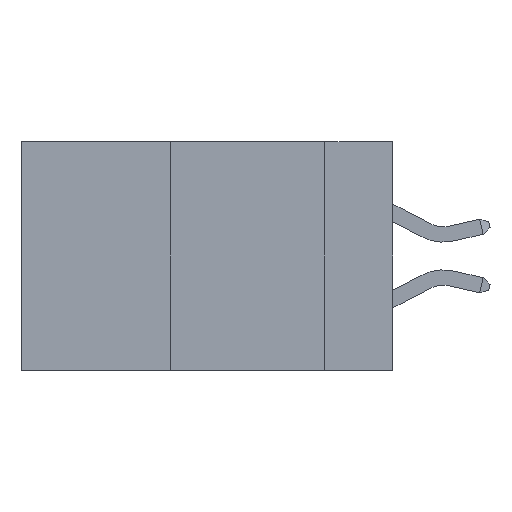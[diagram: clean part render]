
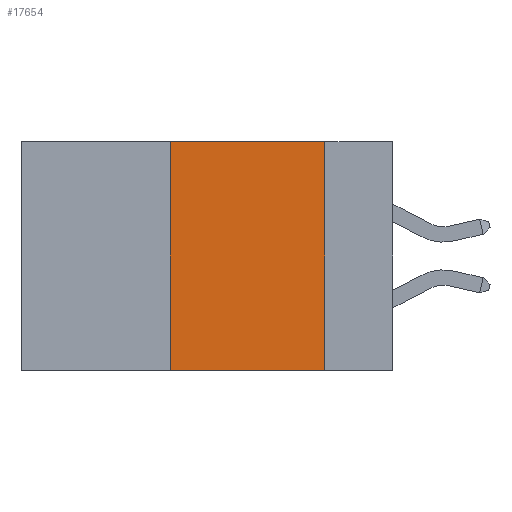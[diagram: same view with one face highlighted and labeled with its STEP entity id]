
A CAD part, left-side view. The second image highlights one B-rep face of the part: STEP entity #17654.
In plain terms, the highlighted planar face has unit normal (-1, 0, 0).
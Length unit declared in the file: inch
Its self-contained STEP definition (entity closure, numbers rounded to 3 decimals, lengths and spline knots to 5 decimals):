
#61 = VECTOR ( 'NONE', #3347, 39.37008 ) ;
#445 = VERTEX_POINT ( 'NONE', #15771 ) ;
#2570 = LINE ( 'NONE', #3486, #11420 ) ;
#2935 = LINE ( 'NONE', #18096, #22303 ) ;
#3347 = DIRECTION ( 'NONE',  ( 0., -1., 0. ) ) ;
#3371 = VERTEX_POINT ( 'NONE', #9484 ) ;
#3486 = CARTESIAN_POINT ( 'NONE',  ( 0., 0.36, 0. ) ) ;
#4096 = DIRECTION ( 'NONE',  ( 1., 0., 0. ) ) ;
#4236 = CARTESIAN_POINT ( 'NONE',  ( 0., 0.36, -0.37 ) ) ;
#5458 = DIRECTION ( 'NONE',  ( 0., -1., 0. ) ) ;
#6753 = EDGE_CURVE ( 'NONE', #15544, #3371, #2570, .T. ) ;
#8447 = VECTOR ( 'NONE', #15380, 39.37008 ) ;
#9484 = CARTESIAN_POINT ( 'NONE',  ( 0., 0.36, 0. ) ) ;
#10056 = LINE ( 'NONE', #10466, #61 ) ;
#10466 = CARTESIAN_POINT ( 'NONE',  ( 0., 0.6, 0. ) ) ;
#11224 = DIRECTION ( 'NONE',  ( 0., 0., -1. ) ) ;
#11420 = VECTOR ( 'NONE', #21050, 39.37008 ) ;
#11885 = VERTEX_POINT ( 'NONE', #21344 ) ;
#12050 = ORIENTED_EDGE ( 'NONE', *, *, #13379, .F. ) ;
#12863 = ORIENTED_EDGE ( 'NONE', *, *, #19494, .T. ) ;
#13198 = CARTESIAN_POINT ( 'NONE',  ( 0., 0.6, 0. ) ) ;
#13379 = EDGE_CURVE ( 'NONE', #3371, #11885, #10056, .T. ) ;
#14546 = LINE ( 'NONE', #15526, #8447 ) ;
#14618 = ORIENTED_EDGE ( 'NONE', *, *, #6753, .F. ) ;
#15350 = AXIS2_PLACEMENT_3D ( 'NONE', #13198, #4096, #11224 ) ;
#15380 = DIRECTION ( 'NONE',  ( 0., 0., -1. ) ) ;
#15526 = CARTESIAN_POINT ( 'NONE',  ( 0., 0.11, 0. ) ) ;
#15544 = VERTEX_POINT ( 'NONE', #4236 ) ;
#15771 = CARTESIAN_POINT ( 'NONE',  ( 0., 0.11, -0.37 ) ) ;
#17654 = ADVANCED_FACE ( 'NONE', ( #19917 ), #20117, .F. ) ;
#18096 = CARTESIAN_POINT ( 'NONE',  ( 0., 0.6, -0.37 ) ) ;
#19494 = EDGE_CURVE ( 'NONE', #15544, #445, #2935, .T. ) ;
#19917 = FACE_OUTER_BOUND ( 'NONE', #21060, .T. ) ;
#20117 = PLANE ( 'NONE',  #15350 ) ;
#20258 = EDGE_CURVE ( 'NONE', #11885, #445, #14546, .T. ) ;
#21050 = DIRECTION ( 'NONE',  ( 0., 0., 1. ) ) ;
#21060 = EDGE_LOOP ( 'NONE', ( #22550, #12050, #14618, #12863 ) ) ;
#21344 = CARTESIAN_POINT ( 'NONE',  ( 0., 0.11, 0. ) ) ;
#22303 = VECTOR ( 'NONE', #5458, 39.37008 ) ;
#22550 = ORIENTED_EDGE ( 'NONE', *, *, #20258, .F. ) ;
